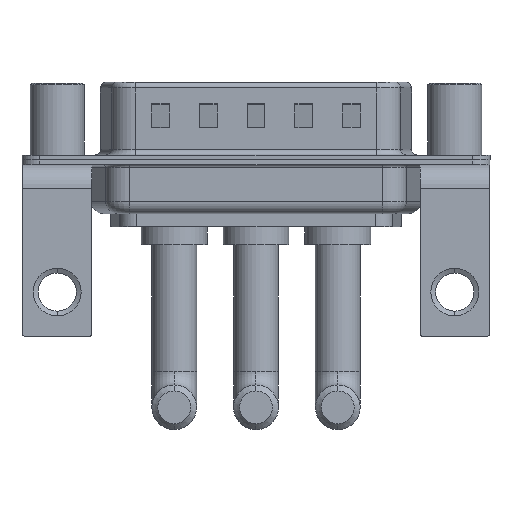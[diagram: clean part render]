
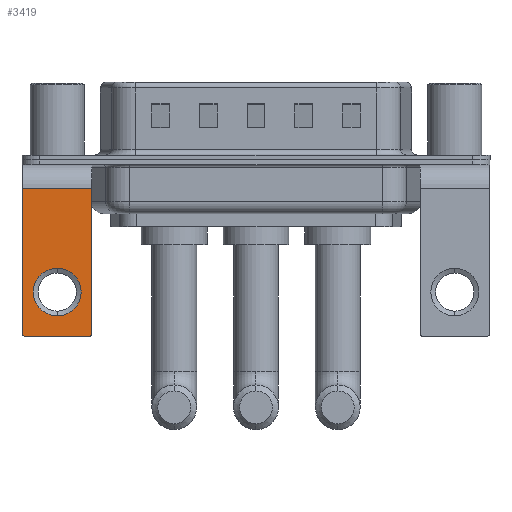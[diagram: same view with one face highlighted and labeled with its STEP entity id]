
A CAD part, front view. The second image highlights one B-rep face of the part: STEP entity #3419.
In plain terms, the highlighted planar face has unit normal (0, -1, 0).
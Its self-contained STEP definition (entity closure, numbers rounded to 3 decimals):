
#489 = DIRECTION ( 'NONE',  ( 0., 1., 0. ) ) ;
#532 = VERTEX_POINT ( 'NONE', #5798 ) ;
#630 = CIRCLE ( 'NONE', #5048, 0.25 ) ;
#1367 = AXIS2_PLACEMENT_3D ( 'NONE', #11964, #17577, #10585 ) ;
#1601 = LINE ( 'NONE', #3145, #14770 ) ;
#1736 = EDGE_CURVE ( 'NONE', #7203, #10248, #4993, .T. ) ;
#1787 = PLANE ( 'NONE',  #2047 ) ;
#2047 = AXIS2_PLACEMENT_3D ( 'NONE', #7415, #6569, #17800 ) ;
#2197 = DIRECTION ( 'NONE',  ( -1., 0., 0. ) ) ;
#2559 = CARTESIAN_POINT ( 'NONE',  ( -2.65, -6.25, -14.8 ) ) ;
#3145 = CARTESIAN_POINT ( 'NONE',  ( 2.9, -6.25, -2.4 ) ) ;
#3419 = ADVANCED_FACE ( 'NONE', ( #5946, #4552 ), #1787, .F. ) ;
#3605 = AXIS2_PLACEMENT_3D ( 'NONE', #6055, #6482, #5291 ) ;
#3696 = VECTOR ( 'NONE', #12666, 1000. ) ;
#4208 = DIRECTION ( 'NONE',  ( 0., -1., 0. ) ) ;
#4547 = EDGE_CURVE ( 'NONE', #6312, #13353, #630, .T. ) ;
#4552 = FACE_OUTER_BOUND ( 'NONE', #9566, .T. ) ;
#4993 = CIRCLE ( 'NONE', #14706, 2. ) ;
#5048 = AXIS2_PLACEMENT_3D ( 'NONE', #11104, #4208, #16737 ) ;
#5136 = EDGE_CURVE ( 'NONE', #8557, #16499, #1601, .T. ) ;
#5291 = DIRECTION ( 'NONE',  ( 0., 0., 1. ) ) ;
#5489 = ORIENTED_EDGE ( 'NONE', *, *, #7957, .T. ) ;
#5798 = CARTESIAN_POINT ( 'NONE',  ( -2.9, -6.25, -14.55 ) ) ;
#5913 = CARTESIAN_POINT ( 'NONE',  ( -2.9, -6.25, -2.4 ) ) ;
#5946 = FACE_BOUND ( 'NONE', #12550, .T. ) ;
#6055 = CARTESIAN_POINT ( 'NONE',  ( -2.65, -6.25, -14.55 ) ) ;
#6255 = LINE ( 'NONE', #5913, #14917 ) ;
#6311 = EDGE_CURVE ( 'NONE', #532, #17716, #12740, .T. ) ;
#6312 = VERTEX_POINT ( 'NONE', #14787 ) ;
#6482 = DIRECTION ( 'NONE',  ( 0., -1., 0. ) ) ;
#6569 = DIRECTION ( 'NONE',  ( 0., 1., 0. ) ) ;
#7203 = VERTEX_POINT ( 'NONE', #16739 ) ;
#7384 = DIRECTION ( 'NONE',  ( 0., 0., -1. ) ) ;
#7394 = DIRECTION ( 'NONE',  ( -1., 0., 0. ) ) ;
#7415 = CARTESIAN_POINT ( 'NONE',  ( 2.9, -6.25, -2.4 ) ) ;
#7922 = LINE ( 'NONE', #13552, #12285 ) ;
#7957 = EDGE_CURVE ( 'NONE', #10248, #7203, #13127, .T. ) ;
#8557 = VERTEX_POINT ( 'NONE', #16454 ) ;
#8967 = EDGE_CURVE ( 'NONE', #8557, #13353, #14316, .T. ) ;
#9566 = EDGE_LOOP ( 'NONE', ( #17931, #12774, #10649, #16953, #16056, #16050 ) ) ;
#10248 = VERTEX_POINT ( 'NONE', #12388 ) ;
#10253 = DIRECTION ( 'NONE',  ( 0., 0., 1. ) ) ;
#10585 = DIRECTION ( 'NONE',  ( 0., 0., 1. ) ) ;
#10649 = ORIENTED_EDGE ( 'NONE', *, *, #13249, .F. ) ;
#11082 = CARTESIAN_POINT ( 'NONE',  ( -2.9, -6.25, -2.4 ) ) ;
#11104 = CARTESIAN_POINT ( 'NONE',  ( 2.65, -6.25, -14.55 ) ) ;
#11416 = ORIENTED_EDGE ( 'NONE', *, *, #1736, .T. ) ;
#11964 = CARTESIAN_POINT ( 'NONE',  ( 0., -6.25, -11.07 ) ) ;
#12285 = VECTOR ( 'NONE', #2197, 1000. ) ;
#12388 = CARTESIAN_POINT ( 'NONE',  ( 0., -6.25, -13.07 ) ) ;
#12550 = EDGE_LOOP ( 'NONE', ( #5489, #11416 ) ) ;
#12666 = DIRECTION ( 'NONE',  ( 0., 0., -1. ) ) ;
#12740 = CIRCLE ( 'NONE', #3605, 0.25 ) ;
#12774 = ORIENTED_EDGE ( 'NONE', *, *, #6311, .T. ) ;
#12779 = EDGE_CURVE ( 'NONE', #16499, #532, #6255, .T. ) ;
#13127 = CIRCLE ( 'NONE', #1367, 2. ) ;
#13249 = EDGE_CURVE ( 'NONE', #6312, #17716, #7922, .T. ) ;
#13353 = VERTEX_POINT ( 'NONE', #18060 ) ;
#13552 = CARTESIAN_POINT ( 'NONE',  ( 2.9, -6.25, -14.8 ) ) ;
#14316 = LINE ( 'NONE', #16985, #3696 ) ;
#14706 = AXIS2_PLACEMENT_3D ( 'NONE', #16052, #489, #10253 ) ;
#14770 = VECTOR ( 'NONE', #7394, 1000. ) ;
#14787 = CARTESIAN_POINT ( 'NONE',  ( 2.65, -6.25, -14.8 ) ) ;
#14917 = VECTOR ( 'NONE', #7384, 1000. ) ;
#16050 = ORIENTED_EDGE ( 'NONE', *, *, #5136, .T. ) ;
#16052 = CARTESIAN_POINT ( 'NONE',  ( 0., -6.25, -11.07 ) ) ;
#16056 = ORIENTED_EDGE ( 'NONE', *, *, #8967, .F. ) ;
#16454 = CARTESIAN_POINT ( 'NONE',  ( 2.9, -6.25, -2.4 ) ) ;
#16499 = VERTEX_POINT ( 'NONE', #11082 ) ;
#16737 = DIRECTION ( 'NONE',  ( 0., 0., 1. ) ) ;
#16739 = CARTESIAN_POINT ( 'NONE',  ( 0., -6.25, -9.07 ) ) ;
#16953 = ORIENTED_EDGE ( 'NONE', *, *, #4547, .T. ) ;
#16985 = CARTESIAN_POINT ( 'NONE',  ( 2.9, -6.25, -2.4 ) ) ;
#17577 = DIRECTION ( 'NONE',  ( 0., 1., 0. ) ) ;
#17716 = VERTEX_POINT ( 'NONE', #2559 ) ;
#17800 = DIRECTION ( 'NONE',  ( 0., 0., 1. ) ) ;
#17931 = ORIENTED_EDGE ( 'NONE', *, *, #12779, .T. ) ;
#18060 = CARTESIAN_POINT ( 'NONE',  ( 2.9, -6.25, -14.55 ) ) ;
